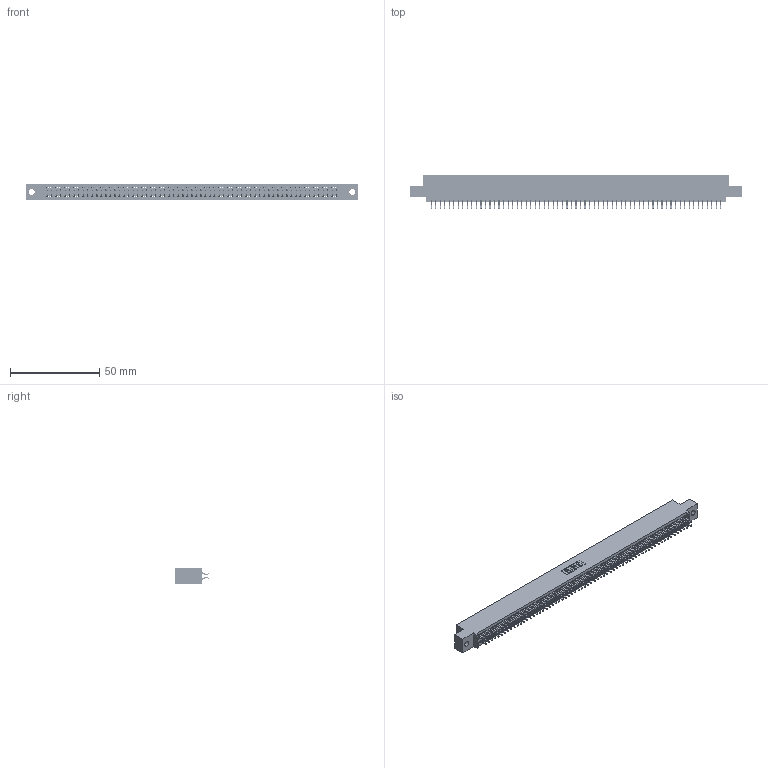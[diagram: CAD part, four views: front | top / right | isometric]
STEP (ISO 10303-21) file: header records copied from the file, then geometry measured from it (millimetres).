
FILE_DESCRIPTION (( 'STEP AP203' ), '1' );
FILE_NAME ('395-130-556-502.STEP', '2018-12-04T19:20:00', ( '' ), ( '' ), 'SwSTEP 2.0', 'SolidWorks 2016', '' );
FILE_SCHEMA (( 'CONFIG_CONTROL_DESIGN' ));
Length unit declared in the file: inch
Products named in the file (3): 345-292-001_556 Tail; 345 Part_0.110 Offset - 0.128 Dia; 395-130-556-502
Assembly tree (131 placements, depth 2):
  395-130-556-502
    345 Part_0.110 Offset - 0.128 Dia
    345-292-001_556 Tail  x130
Bounding box: 186.31 x 19.24 x 9.4 mm (x, y, z)
Volume: 18196.5 mm3; surface area: 27049.3 mm2
Topology: 131 solids, 131 shells, 7410 faces, 22063 edges, 14534 vertices
Faces by surface type: plane 4894, cylinder 2516
Entity records: 48259 total; most frequent: CARTESIAN_POINT 8084, ORIENTED_EDGE 8006, DIRECTION 7087, EDGE_CURVE 4003, VECTOR 3603, LINE 3603, VERTEX_POINT 2666, AXIS2_PLACEMENT_3D 1742
